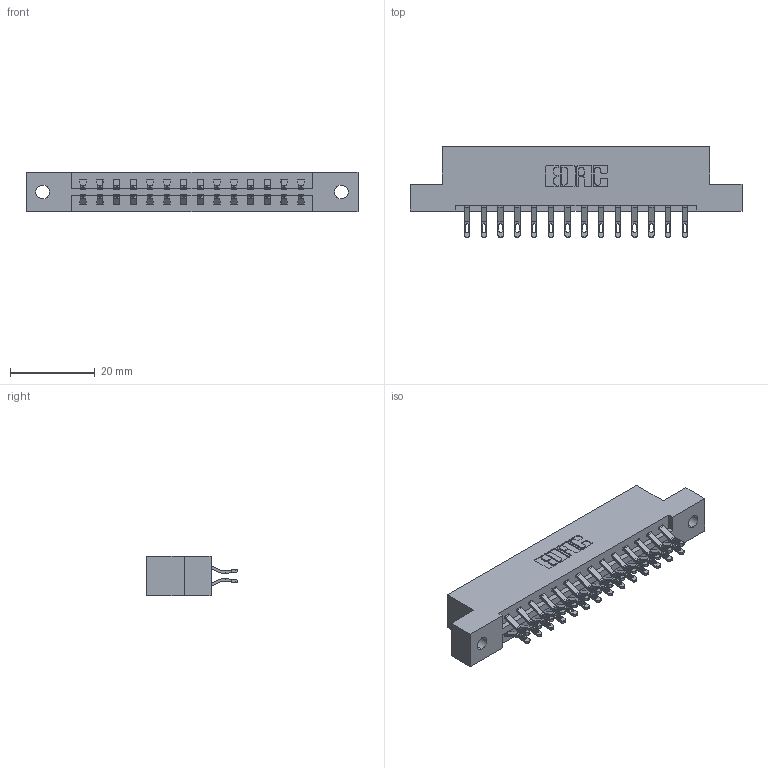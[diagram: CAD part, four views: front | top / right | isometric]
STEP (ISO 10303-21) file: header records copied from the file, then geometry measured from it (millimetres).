
FILE_DESCRIPTION (( 'STEP AP203' ), '1' );
FILE_NAME ('337-028-555-202.STEP', '2018-08-06T11:37:48', ( '' ), ( '' ), 'SwSTEP 2.0', 'SolidWorks 2016', '' );
FILE_SCHEMA (( 'CONFIG_CONTROL_DESIGN' ));
Length unit declared in the file: inch
Products named in the file (3): 337-028-555-202; 337 Part_Flush Mounting Lugs - 0.128 Dia; 345-292-001_555 Tail
Assembly tree (29 placements, depth 2):
  337-028-555-202
    337 Part_Flush Mounting Lugs - 0.128 Dia
    345-292-001_555 Tail  x28
Bounding box: 78.49 x 21.47 x 9.4 mm (x, y, z)
Volume: 7943.3 mm3; surface area: 8741.3 mm2
Topology: 29 solids, 29 shells, 1794 faces, 5603 edges, 3734 vertices
Faces by surface type: plane 1078, cylinder 716
Entity records: 14805 total; most frequent: CARTESIAN_POINT 2552, ORIENTED_EDGE 2458, DIRECTION 2193, EDGE_CURVE 1229, LINE 1081, VECTOR 1081, VERTEX_POINT 818, AXIS2_PLACEMENT_3D 556
